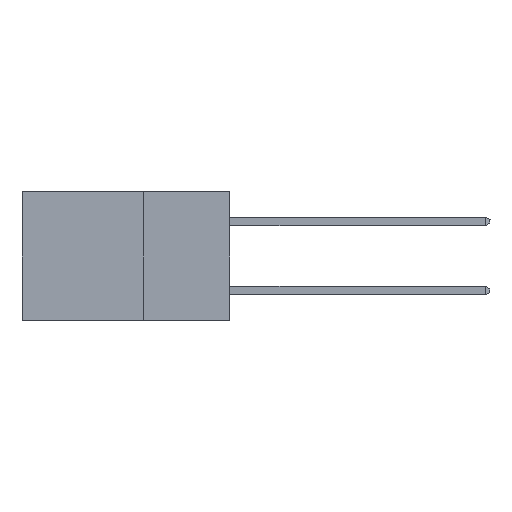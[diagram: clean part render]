
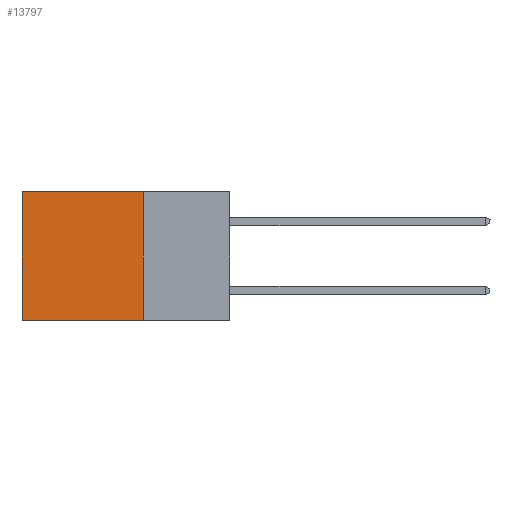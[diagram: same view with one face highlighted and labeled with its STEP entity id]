
A CAD part, left-side view. The second image highlights one B-rep face of the part: STEP entity #13797.
In plain terms, the highlighted planar face has unit normal (-1, 0, 0).
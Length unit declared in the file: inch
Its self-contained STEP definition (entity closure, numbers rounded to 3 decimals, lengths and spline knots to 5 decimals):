
#140 = VECTOR ( 'NONE', #13384, 39.37008 ) ;
#449 = CARTESIAN_POINT ( 'NONE',  ( 0.2615, 0.25, -0.37 ) ) ;
#489 = CARTESIAN_POINT ( 'NONE',  ( 0.2615, 0.25, -0.37 ) ) ;
#540 = CARTESIAN_POINT ( 'NONE',  ( 0.2615, 0.6, -0.37 ) ) ;
#542 = EDGE_CURVE ( 'NONE', #11532, #11337, #13454, .T. ) ;
#1125 = ORIENTED_EDGE ( 'NONE', *, *, #14259, .T. ) ;
#1332 = VECTOR ( 'NONE', #7046, 39.37008 ) ;
#1812 = FACE_OUTER_BOUND ( 'NONE', #2451, .T. ) ;
#2070 = VERTEX_POINT ( 'NONE', #7272 ) ;
#2451 = EDGE_LOOP ( 'NONE', ( #11192, #16356, #5167, #1125 ) ) ;
#2676 = VECTOR ( 'NONE', #9400, 39.37008 ) ;
#4279 = CARTESIAN_POINT ( 'NONE',  ( 0.2615, 0.6, -0.37 ) ) ;
#5167 = ORIENTED_EDGE ( 'NONE', *, *, #16354, .F. ) ;
#5904 = CARTESIAN_POINT ( 'NONE',  ( 0.2615, 0.25, 0. ) ) ;
#6931 = DIRECTION ( 'NONE',  ( 1., 0., 0. ) ) ;
#7046 = DIRECTION ( 'NONE',  ( 0., 1., 0. ) ) ;
#7272 = CARTESIAN_POINT ( 'NONE',  ( 0.2615, 0.6, 0. ) ) ;
#7685 = EDGE_CURVE ( 'NONE', #2070, #11337, #9664, .T. ) ;
#8028 = VERTEX_POINT ( 'NONE', #9563 ) ;
#8116 = AXIS2_PLACEMENT_3D ( 'NONE', #489, #6931, #11895 ) ;
#8432 = VECTOR ( 'NONE', #9137, 39.37008 ) ;
#8676 = CARTESIAN_POINT ( 'NONE',  ( 0.2615, 0.25, -0.37 ) ) ;
#9137 = DIRECTION ( 'NONE',  ( 0., 0., -1. ) ) ;
#9400 = DIRECTION ( 'NONE',  ( 0., 0., -1. ) ) ;
#9563 = CARTESIAN_POINT ( 'NONE',  ( 0.2615, 0.25, 0. ) ) ;
#9601 = LINE ( 'NONE', #5904, #140 ) ;
#9664 = LINE ( 'NONE', #4279, #2676 ) ;
#11192 = ORIENTED_EDGE ( 'NONE', *, *, #7685, .T. ) ;
#11337 = VERTEX_POINT ( 'NONE', #540 ) ;
#11507 = LINE ( 'NONE', #15534, #8432 ) ;
#11532 = VERTEX_POINT ( 'NONE', #8676 ) ;
#11895 = DIRECTION ( 'NONE',  ( 0., 0., -1. ) ) ;
#13384 = DIRECTION ( 'NONE',  ( 0., 1., 0. ) ) ;
#13454 = LINE ( 'NONE', #449, #1332 ) ;
#13797 = ADVANCED_FACE ( 'NONE', ( #1812 ), #16290, .F. ) ;
#14259 = EDGE_CURVE ( 'NONE', #8028, #2070, #9601, .T. ) ;
#15534 = CARTESIAN_POINT ( 'NONE',  ( 0.2615, 0.25, -0.37 ) ) ;
#16290 = PLANE ( 'NONE',  #8116 ) ;
#16354 = EDGE_CURVE ( 'NONE', #8028, #11532, #11507, .T. ) ;
#16356 = ORIENTED_EDGE ( 'NONE', *, *, #542, .F. ) ;
